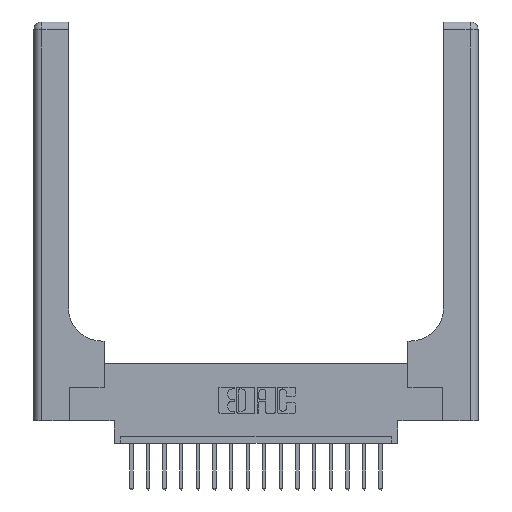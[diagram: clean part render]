
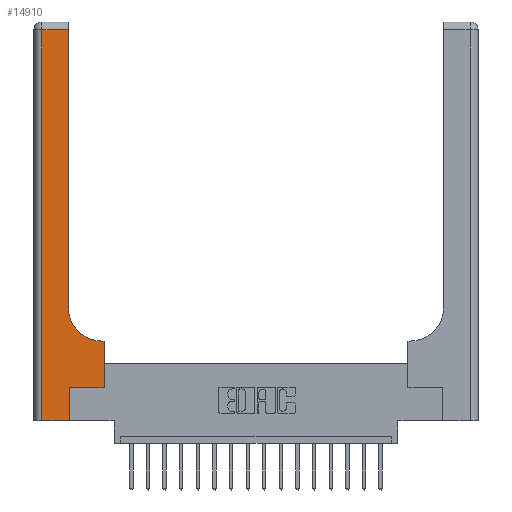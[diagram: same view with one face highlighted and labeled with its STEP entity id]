
A CAD part, top view. The second image highlights one B-rep face of the part: STEP entity #14910.
In plain terms, the highlighted planar face has unit normal (0, 0, 1).
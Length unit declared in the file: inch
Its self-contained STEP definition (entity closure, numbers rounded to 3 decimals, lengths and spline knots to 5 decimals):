
#42 = CARTESIAN_POINT ( 'NONE',  ( 0.265, 0., 0.37 ) ) ;
#267 = CARTESIAN_POINT ( 'NONE',  ( 0.51, 0.85, 0.37 ) ) ;
#380 = VERTEX_POINT ( 'NONE', #5841 ) ;
#429 = VERTEX_POINT ( 'NONE', #8606 ) ;
#961 = VERTEX_POINT ( 'NONE', #14844 ) ;
#1186 = VECTOR ( 'NONE', #14137, 39.37008 ) ;
#1416 = DIRECTION ( 'NONE',  ( -1., 0., 0. ) ) ;
#1718 = ORIENTED_EDGE ( 'NONE', *, *, #9518, .T. ) ;
#1852 = CARTESIAN_POINT ( 'NONE',  ( 0.51, 0.6, 0.37 ) ) ;
#1931 = CARTESIAN_POINT ( 'NONE',  ( 0.26, 3., 0.37 ) ) ;
#2322 = VERTEX_POINT ( 'NONE', #42 ) ;
#2978 = CARTESIAN_POINT ( 'NONE',  ( 0., 3., 0.37 ) ) ;
#3044 = DIRECTION ( 'NONE',  ( 1., 0., 0. ) ) ;
#3207 = ORIENTED_EDGE ( 'NONE', *, *, #3882, .T. ) ;
#3240 = ORIENTED_EDGE ( 'NONE', *, *, #6498, .T. ) ;
#3411 = VERTEX_POINT ( 'NONE', #9620 ) ;
#3465 = LINE ( 'NONE', #16954, #1186 ) ;
#3565 = DIRECTION ( 'NONE',  ( 1., 0., 0. ) ) ;
#3787 = CARTESIAN_POINT ( 'NONE',  ( 0.265, 0.25, 0.37 ) ) ;
#3882 = EDGE_CURVE ( 'NONE', #17394, #961, #8917, .T. ) ;
#4131 = LINE ( 'NONE', #12285, #14354 ) ;
#5160 = ORIENTED_EDGE ( 'NONE', *, *, #14403, .T. ) ;
#5522 = CARTESIAN_POINT ( 'NONE',  ( 0.06, 0., 0.37 ) ) ;
#5841 = CARTESIAN_POINT ( 'NONE',  ( 0.528, 0.25, 0.37 ) ) ;
#5937 = DIRECTION ( 'NONE',  ( 0., 0., -1. ) ) ;
#5999 = VECTOR ( 'NONE', #10690, 39.37008 ) ;
#6081 = EDGE_LOOP ( 'NONE', ( #6917, #3207, #14020, #1718, #8121, #16604, #3240, #14996, #5160 ) ) ;
#6377 = CARTESIAN_POINT ( 'NONE',  ( 0., 0., 0.37 ) ) ;
#6399 = VECTOR ( 'NONE', #11961, 39.37008 ) ;
#6498 = EDGE_CURVE ( 'NONE', #380, #3411, #3465, .T. ) ;
#6558 = DIRECTION ( 'NONE',  ( 1., 0., 0. ) ) ;
#6917 = ORIENTED_EDGE ( 'NONE', *, *, #12483, .T. ) ;
#7025 = AXIS2_PLACEMENT_3D ( 'NONE', #267, #10365, #3044 ) ;
#7223 = VERTEX_POINT ( 'NONE', #1852 ) ;
#7491 = CIRCLE ( 'NONE', #7025, 0.25 ) ;
#7542 = DIRECTION ( 'NONE',  ( 0., 1., 0. ) ) ;
#7690 = LINE ( 'NONE', #9277, #15632 ) ;
#8121 = ORIENTED_EDGE ( 'NONE', *, *, #18236, .T. ) ;
#8606 = CARTESIAN_POINT ( 'NONE',  ( 0.26, 0.85, 0.37 ) ) ;
#8878 = VECTOR ( 'NONE', #7542, 39.37008 ) ;
#8917 = LINE ( 'NONE', #14882, #6399 ) ;
#9277 = CARTESIAN_POINT ( 'NONE',  ( 0.06, 3., 0.37 ) ) ;
#9346 = DIRECTION ( 'NONE',  ( 0., -1., 0. ) ) ;
#9518 = EDGE_CURVE ( 'NONE', #10920, #2322, #15618, .T. ) ;
#9620 = CARTESIAN_POINT ( 'NONE',  ( 0.528, 0.6, 0.37 ) ) ;
#9762 = LINE ( 'NONE', #10401, #8878 ) ;
#10247 = LINE ( 'NONE', #12986, #16156 ) ;
#10365 = DIRECTION ( 'NONE',  ( 0., 0., -1. ) ) ;
#10401 = CARTESIAN_POINT ( 'NONE',  ( 0.265, 0., 0.37 ) ) ;
#10690 = DIRECTION ( 'NONE',  ( 0., 1., 0. ) ) ;
#10920 = VERTEX_POINT ( 'NONE', #5522 ) ;
#10978 = EDGE_CURVE ( 'NONE', #3411, #7223, #10247, .T. ) ;
#11821 = FACE_OUTER_BOUND ( 'NONE', #6081, .T. ) ;
#11961 = DIRECTION ( 'NONE',  ( -1., 0., 0. ) ) ;
#12285 = CARTESIAN_POINT ( 'NONE',  ( 0.265, 0.25, 0.37 ) ) ;
#12483 = EDGE_CURVE ( 'NONE', #429, #17394, #12587, .T. ) ;
#12587 = LINE ( 'NONE', #1931, #5999 ) ;
#12986 = CARTESIAN_POINT ( 'NONE',  ( 0.26, 0.6, 0.37 ) ) ;
#13220 = VERTEX_POINT ( 'NONE', #3787 ) ;
#13433 = EDGE_CURVE ( 'NONE', #13220, #380, #4131, .T. ) ;
#14020 = ORIENTED_EDGE ( 'NONE', *, *, #15190, .T. ) ;
#14137 = DIRECTION ( 'NONE',  ( 0., 1., 0. ) ) ;
#14354 = VECTOR ( 'NONE', #3565, 39.37008 ) ;
#14403 = EDGE_CURVE ( 'NONE', #7223, #429, #7491, .T. ) ;
#14835 = CARTESIAN_POINT ( 'NONE',  ( 0.26, 2.94, 0.37 ) ) ;
#14844 = CARTESIAN_POINT ( 'NONE',  ( 0.06, 2.94, 0.37 ) ) ;
#14882 = CARTESIAN_POINT ( 'NONE',  ( 0., 2.94, 0.37 ) ) ;
#14910 = ADVANCED_FACE ( 'NONE', ( #11821 ), #16136, .F. ) ;
#14968 = AXIS2_PLACEMENT_3D ( 'NONE', #2978, #5937, #1416 ) ;
#14996 = ORIENTED_EDGE ( 'NONE', *, *, #10978, .T. ) ;
#15177 = VECTOR ( 'NONE', #6558, 39.37008 ) ;
#15190 = EDGE_CURVE ( 'NONE', #961, #10920, #7690, .T. ) ;
#15618 = LINE ( 'NONE', #6377, #15177 ) ;
#15632 = VECTOR ( 'NONE', #9346, 39.37008 ) ;
#15828 = DIRECTION ( 'NONE',  ( -1., 0., 0. ) ) ;
#16136 = PLANE ( 'NONE',  #14968 ) ;
#16156 = VECTOR ( 'NONE', #15828, 39.37008 ) ;
#16604 = ORIENTED_EDGE ( 'NONE', *, *, #13433, .T. ) ;
#16954 = CARTESIAN_POINT ( 'NONE',  ( 0.528, 0.25, 0.37 ) ) ;
#17394 = VERTEX_POINT ( 'NONE', #14835 ) ;
#18236 = EDGE_CURVE ( 'NONE', #2322, #13220, #9762, .T. ) ;
